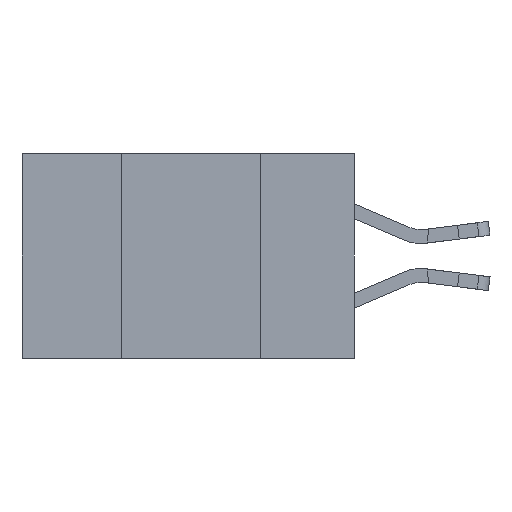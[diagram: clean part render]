
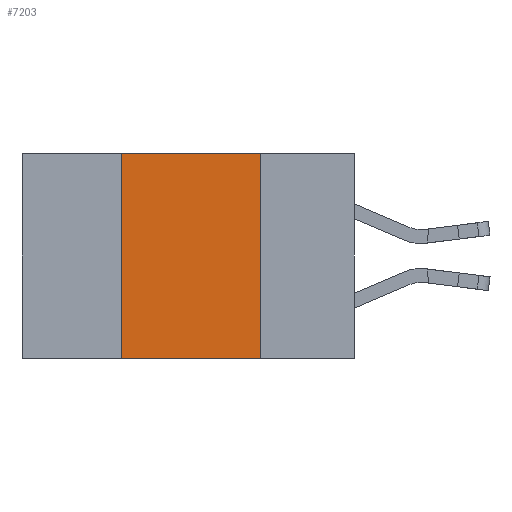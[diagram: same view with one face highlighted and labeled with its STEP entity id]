
A CAD part, left-side view. The second image highlights one B-rep face of the part: STEP entity #7203.
In plain terms, the highlighted planar face has unit normal (-1, 0, 0).
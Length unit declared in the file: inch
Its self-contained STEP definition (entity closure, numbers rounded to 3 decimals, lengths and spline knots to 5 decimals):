
#452 = LINE ( 'NONE', #6655, #4233 ) ;
#502 = VECTOR ( 'NONE', #3077, 39.37008 ) ;
#763 = ORIENTED_EDGE ( 'NONE', *, *, #7564, .T. ) ;
#810 = ORIENTED_EDGE ( 'NONE', *, *, #11555, .F. ) ;
#1131 = VERTEX_POINT ( 'NONE', #10511 ) ;
#1259 = EDGE_CURVE ( 'NONE', #4618, #2851, #9735, .T. ) ;
#1748 = DIRECTION ( 'NONE',  ( 0., -1., 0. ) ) ;
#1762 = CARTESIAN_POINT ( 'NONE',  ( 0., 0.42, 0. ) ) ;
#2814 = FACE_OUTER_BOUND ( 'NONE', #9998, .T. ) ;
#2851 = VERTEX_POINT ( 'NONE', #7059 ) ;
#3077 = DIRECTION ( 'NONE',  ( 0., -1., 0. ) ) ;
#3215 = DIRECTION ( 'NONE',  ( 0., 0., 1. ) ) ;
#3772 = ORIENTED_EDGE ( 'NONE', *, *, #9542, .F. ) ;
#4183 = DIRECTION ( 'NONE',  ( 0., 0., -1. ) ) ;
#4191 = VERTEX_POINT ( 'NONE', #10646 ) ;
#4227 = DIRECTION ( 'NONE',  ( 1., 0., 0. ) ) ;
#4233 = VECTOR ( 'NONE', #5671, 39.37008 ) ;
#4410 = ORIENTED_EDGE ( 'NONE', *, *, #1259, .F. ) ;
#4618 = VERTEX_POINT ( 'NONE', #1762 ) ;
#5671 = DIRECTION ( 'NONE',  ( 0., 0., -1. ) ) ;
#5804 = LINE ( 'NONE', #9742, #10943 ) ;
#5857 = VECTOR ( 'NONE', #1748, 39.37008 ) ;
#6127 = CARTESIAN_POINT ( 'NONE',  ( 0., 0.6, -0.37 ) ) ;
#6655 = CARTESIAN_POINT ( 'NONE',  ( 0., 0.17, 0. ) ) ;
#7059 = CARTESIAN_POINT ( 'NONE',  ( 0., 0.17, 0. ) ) ;
#7203 = ADVANCED_FACE ( 'NONE', ( #2814 ), #11816, .F. ) ;
#7369 = CARTESIAN_POINT ( 'NONE',  ( 0., 0.6, 0. ) ) ;
#7564 = EDGE_CURVE ( 'NONE', #4191, #1131, #12519, .T. ) ;
#9542 = EDGE_CURVE ( 'NONE', #4191, #4618, #5804, .T. ) ;
#9557 = AXIS2_PLACEMENT_3D ( 'NONE', #7369, #4227, #4183 ) ;
#9735 = LINE ( 'NONE', #14098, #502 ) ;
#9742 = CARTESIAN_POINT ( 'NONE',  ( 0., 0.42, 0. ) ) ;
#9998 = EDGE_LOOP ( 'NONE', ( #810, #4410, #3772, #763 ) ) ;
#10511 = CARTESIAN_POINT ( 'NONE',  ( 0., 0.17, -0.37 ) ) ;
#10646 = CARTESIAN_POINT ( 'NONE',  ( 0., 0.42, -0.37 ) ) ;
#10943 = VECTOR ( 'NONE', #3215, 39.37008 ) ;
#11555 = EDGE_CURVE ( 'NONE', #2851, #1131, #452, .T. ) ;
#11816 = PLANE ( 'NONE',  #9557 ) ;
#12519 = LINE ( 'NONE', #6127, #5857 ) ;
#14098 = CARTESIAN_POINT ( 'NONE',  ( 0., 0.6, 0. ) ) ;
